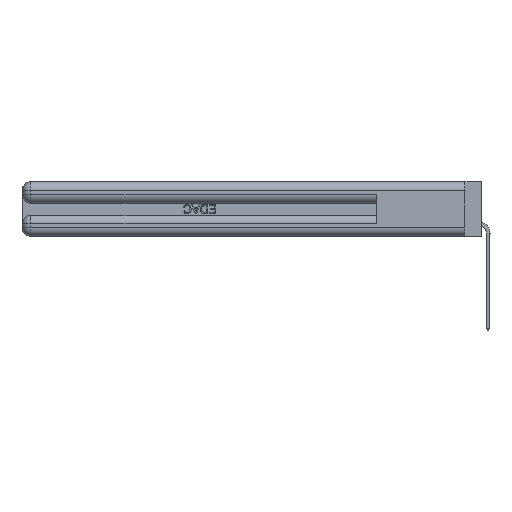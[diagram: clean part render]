
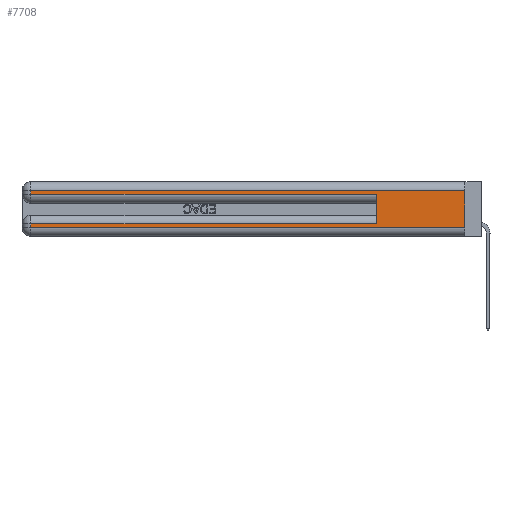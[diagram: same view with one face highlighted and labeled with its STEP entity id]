
A CAD part, left-side view. The second image highlights one B-rep face of the part: STEP entity #7708.
In plain terms, the highlighted planar face has unit normal (-1, 0, 0).
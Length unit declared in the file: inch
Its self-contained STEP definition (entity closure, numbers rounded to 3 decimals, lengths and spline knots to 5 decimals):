
#1028 = DIRECTION ( 'NONE',  ( 1., 0., 0. ) ) ;
#1267 = EDGE_LOOP ( 'NONE', ( #5716, #3229, #10504, #10576, #27786, #34096, #4333, #37648 ) ) ;
#1837 = CARTESIAN_POINT ( 'NONE',  ( 0., 0., 0.31 ) ) ;
#1890 = CARTESIAN_POINT ( 'NONE',  ( 0., 0.6, 0.285 ) ) ;
#2114 = EDGE_CURVE ( 'NONE', #35393, #25588, #9911, .T. ) ;
#3229 = ORIENTED_EDGE ( 'NONE', *, *, #2114, .T. ) ;
#3575 = VECTOR ( 'NONE', #9503, 39.37008 ) ;
#3674 = CARTESIAN_POINT ( 'NONE',  ( 0., 0.6, 0.145 ) ) ;
#4333 = ORIENTED_EDGE ( 'NONE', *, *, #35953, .T. ) ;
#5018 = DIRECTION ( 'NONE',  ( 0., 0., -1. ) ) ;
#5716 = ORIENTED_EDGE ( 'NONE', *, *, #25180, .F. ) ;
#7708 = ADVANCED_FACE ( 'NONE', ( #22711 ), #17670, .F. ) ;
#8033 = VERTEX_POINT ( 'NONE', #1890 ) ;
#9503 = DIRECTION ( 'NONE',  ( 0., 0., 1. ) ) ;
#9911 = LINE ( 'NONE', #29141, #33613 ) ;
#10127 = CARTESIAN_POINT ( 'NONE',  ( 0., 2.94, 0.37 ) ) ;
#10504 = ORIENTED_EDGE ( 'NONE', *, *, #14282, .T. ) ;
#10576 = ORIENTED_EDGE ( 'NONE', *, *, #18349, .T. ) ;
#10986 = LINE ( 'NONE', #16056, #36045 ) ;
#11454 = VECTOR ( 'NONE', #24800, 39.37008 ) ;
#12558 = LINE ( 'NONE', #34632, #24863 ) ;
#12691 = CARTESIAN_POINT ( 'NONE',  ( 0., 0., 0.37 ) ) ;
#13824 = CARTESIAN_POINT ( 'NONE',  ( 0., 0., 0.06 ) ) ;
#14282 = EDGE_CURVE ( 'NONE', #25588, #25226, #12558, .T. ) ;
#14577 = DIRECTION ( 'NONE',  ( 0., 1., 0. ) ) ;
#16056 = CARTESIAN_POINT ( 'NONE',  ( 0., 0., 0.285 ) ) ;
#16125 = AXIS2_PLACEMENT_3D ( 'NONE', #12691, #1028, #35441 ) ;
#16598 = LINE ( 'NONE', #10127, #18848 ) ;
#16674 = DIRECTION ( 'NONE',  ( 0., -1., 0. ) ) ;
#17337 = CARTESIAN_POINT ( 'NONE',  ( 0., 2.94, 0.31 ) ) ;
#17461 = CARTESIAN_POINT ( 'NONE',  ( 0., 2.94, 0.285 ) ) ;
#17670 = PLANE ( 'NONE',  #16125 ) ;
#18148 = VERTEX_POINT ( 'NONE', #13824 ) ;
#18349 = EDGE_CURVE ( 'NONE', #25226, #8033, #10986, .T. ) ;
#18848 = VECTOR ( 'NONE', #21730, 39.37008 ) ;
#20358 = EDGE_CURVE ( 'NONE', #37053, #8033, #36344, .T. ) ;
#20479 = DIRECTION ( 'NONE',  ( 0., 1., 0. ) ) ;
#20617 = CARTESIAN_POINT ( 'NONE',  ( 0., 0.6, 0.085 ) ) ;
#21006 = VECTOR ( 'NONE', #5018, 39.37008 ) ;
#21730 = DIRECTION ( 'NONE',  ( 0., 0., -1. ) ) ;
#22568 = CARTESIAN_POINT ( 'NONE',  ( 0., 2.94, 0.06 ) ) ;
#22711 = FACE_OUTER_BOUND ( 'NONE', #1267, .T. ) ;
#24709 = VECTOR ( 'NONE', #20479, 39.37008 ) ;
#24800 = DIRECTION ( 'NONE',  ( 0., -1., 0. ) ) ;
#24863 = VECTOR ( 'NONE', #37059, 39.37008 ) ;
#25180 = EDGE_CURVE ( 'NONE', #35393, #18148, #28744, .T. ) ;
#25226 = VERTEX_POINT ( 'NONE', #17461 ) ;
#25588 = VERTEX_POINT ( 'NONE', #17337 ) ;
#26371 = VERTEX_POINT ( 'NONE', #36529 ) ;
#27786 = ORIENTED_EDGE ( 'NONE', *, *, #20358, .F. ) ;
#28744 = LINE ( 'NONE', #31054, #21006 ) ;
#29141 = CARTESIAN_POINT ( 'NONE',  ( 0., 0., 0.31 ) ) ;
#31054 = CARTESIAN_POINT ( 'NONE',  ( 0., 0., 0.37 ) ) ;
#32283 = EDGE_CURVE ( 'NONE', #37053, #26371, #36992, .T. ) ;
#32838 = LINE ( 'NONE', #33193, #11454 ) ;
#32953 = EDGE_CURVE ( 'NONE', #37309, #18148, #32838, .T. ) ;
#33193 = CARTESIAN_POINT ( 'NONE',  ( 0., 0., 0.06 ) ) ;
#33613 = VECTOR ( 'NONE', #14577, 39.37008 ) ;
#34096 = ORIENTED_EDGE ( 'NONE', *, *, #32283, .T. ) ;
#34632 = CARTESIAN_POINT ( 'NONE',  ( 0., 2.94, 0.37 ) ) ;
#34980 = CARTESIAN_POINT ( 'NONE',  ( 0., 0., 0.085 ) ) ;
#35393 = VERTEX_POINT ( 'NONE', #1837 ) ;
#35441 = DIRECTION ( 'NONE',  ( 0., 0., -1. ) ) ;
#35953 = EDGE_CURVE ( 'NONE', #26371, #37309, #16598, .T. ) ;
#36045 = VECTOR ( 'NONE', #16674, 39.37008 ) ;
#36344 = LINE ( 'NONE', #3674, #3575 ) ;
#36529 = CARTESIAN_POINT ( 'NONE',  ( 0., 2.94, 0.085 ) ) ;
#36992 = LINE ( 'NONE', #34980, #24709 ) ;
#37053 = VERTEX_POINT ( 'NONE', #20617 ) ;
#37059 = DIRECTION ( 'NONE',  ( 0., 0., -1. ) ) ;
#37309 = VERTEX_POINT ( 'NONE', #22568 ) ;
#37648 = ORIENTED_EDGE ( 'NONE', *, *, #32953, .T. ) ;
